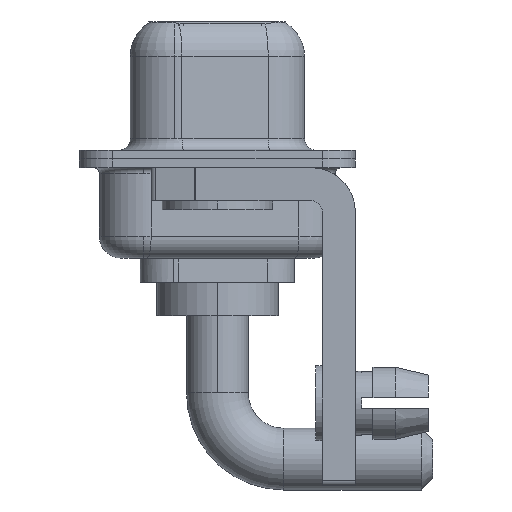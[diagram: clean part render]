
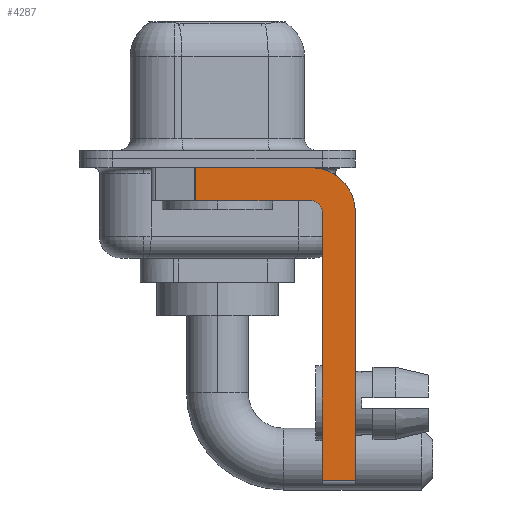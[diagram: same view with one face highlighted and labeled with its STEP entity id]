
A CAD part, left-side view. The second image highlights one B-rep face of the part: STEP entity #4287.
In plain terms, the highlighted planar face has unit normal (-1, 0, 0).
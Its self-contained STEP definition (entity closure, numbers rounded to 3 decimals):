
#157 = DIRECTION ( 'NONE',  ( -1., 0., 0. ) ) ;
#300 = DIRECTION ( 'NONE',  ( 0., -1., 0. ) ) ;
#726 = CARTESIAN_POINT ( 'NONE',  ( -2.9, 0.978, -1.9 ) ) ;
#1326 = ORIENTED_EDGE ( 'NONE', *, *, #11066, .F. ) ;
#1435 = EDGE_CURVE ( 'NONE', #13794, #10026, #7171, .T. ) ;
#1585 = EDGE_CURVE ( 'NONE', #13017, #10026, #4203, .T. ) ;
#1808 = DIRECTION ( 'NONE',  ( 1., 0., 0. ) ) ;
#1882 = EDGE_CURVE ( 'NONE', #11429, #8898, #6978, .T. ) ;
#1981 = CARTESIAN_POINT ( 'NONE',  ( -2.9, -4.75, -2.4 ) ) ;
#2211 = AXIS2_PLACEMENT_3D ( 'NONE', #14716, #1808, #3368 ) ;
#2222 = CIRCLE ( 'NONE', #2211, 2. ) ;
#2811 = DIRECTION ( 'NONE',  ( 0., 0., 1. ) ) ;
#2895 = CARTESIAN_POINT ( 'NONE',  ( -2.9, -4.25, -1.9 ) ) ;
#3368 = DIRECTION ( 'NONE',  ( 0., 0., -1. ) ) ;
#3976 = CARTESIAN_POINT ( 'NONE',  ( -2.9, -6.25, -2.4 ) ) ;
#4047 = DIRECTION ( 'NONE',  ( 0., 0., -1. ) ) ;
#4203 = LINE ( 'NONE', #12189, #13978 ) ;
#4283 = DIRECTION ( 'NONE',  ( 0., 0., -1. ) ) ;
#4287 = ADVANCED_FACE ( 'NONE', ( #6361 ), #8532, .F. ) ;
#4572 = CIRCLE ( 'NONE', #12906, 0.5 ) ;
#4833 = DIRECTION ( 'NONE',  ( 0., 1., 0. ) ) ;
#4939 = LINE ( 'NONE', #7006, #14163 ) ;
#4946 = ORIENTED_EDGE ( 'NONE', *, *, #11158, .F. ) ;
#4957 = ORIENTED_EDGE ( 'NONE', *, *, #8783, .F. ) ;
#4991 = ORIENTED_EDGE ( 'NONE', *, *, #1435, .F. ) ;
#5281 = AXIS2_PLACEMENT_3D ( 'NONE', #8834, #14218, #4283 ) ;
#5479 = EDGE_CURVE ( 'NONE', #8680, #8898, #11566, .T. ) ;
#6321 = EDGE_LOOP ( 'NONE', ( #4946, #8584, #10918, #7798, #4957, #13199, #4991, #1326 ) ) ;
#6361 = FACE_OUTER_BOUND ( 'NONE', #6321, .T. ) ;
#6978 = LINE ( 'NONE', #13871, #12560 ) ;
#7006 = CARTESIAN_POINT ( 'NONE',  ( -2.9, 3., -0.4 ) ) ;
#7130 = CARTESIAN_POINT ( 'NONE',  ( -2.9, 0.978, -1.9 ) ) ;
#7171 = LINE ( 'NONE', #3976, #7762 ) ;
#7762 = VECTOR ( 'NONE', #4047, 1000. ) ;
#7798 = ORIENTED_EDGE ( 'NONE', *, *, #8747, .F. ) ;
#8532 = PLANE ( 'NONE',  #5281 ) ;
#8584 = ORIENTED_EDGE ( 'NONE', *, *, #5479, .T. ) ;
#8680 = VERTEX_POINT ( 'NONE', #10447 ) ;
#8747 = EDGE_CURVE ( 'NONE', #11525, #11429, #4572, .T. ) ;
#8783 = EDGE_CURVE ( 'NONE', #13017, #11525, #10591, .T. ) ;
#8834 = CARTESIAN_POINT ( 'NONE',  ( -2.9, -4.25, -2.4 ) ) ;
#8898 = VERTEX_POINT ( 'NONE', #726 ) ;
#9259 = DIRECTION ( 'NONE',  ( 0., 0., 1. ) ) ;
#9473 = CARTESIAN_POINT ( 'NONE',  ( -2.9, -4.75, -14.8 ) ) ;
#9536 = VECTOR ( 'NONE', #2811, 1000. ) ;
#9962 = CARTESIAN_POINT ( 'NONE',  ( -2.9, -6.25, -2.4 ) ) ;
#10026 = VERTEX_POINT ( 'NONE', #11690 ) ;
#10447 = CARTESIAN_POINT ( 'NONE',  ( -2.9, 0.978, -0.4 ) ) ;
#10471 = VECTOR ( 'NONE', #10576, 1000. ) ;
#10576 = DIRECTION ( 'NONE',  ( 0., 0., -1. ) ) ;
#10591 = LINE ( 'NONE', #9473, #9536 ) ;
#10670 = CARTESIAN_POINT ( 'NONE',  ( -2.9, -4.25, -2.4 ) ) ;
#10918 = ORIENTED_EDGE ( 'NONE', *, *, #1882, .F. ) ;
#11066 = EDGE_CURVE ( 'NONE', #12362, #13794, #2222, .T. ) ;
#11158 = EDGE_CURVE ( 'NONE', #8680, #12362, #4939, .T. ) ;
#11425 = DIRECTION ( 'NONE',  ( 0., -1., 0. ) ) ;
#11429 = VERTEX_POINT ( 'NONE', #2895 ) ;
#11525 = VERTEX_POINT ( 'NONE', #1981 ) ;
#11566 = LINE ( 'NONE', #7130, #10471 ) ;
#11690 = CARTESIAN_POINT ( 'NONE',  ( -2.9, -6.25, -14.55 ) ) ;
#12189 = CARTESIAN_POINT ( 'NONE',  ( -2.9, -4.25, -14.55 ) ) ;
#12362 = VERTEX_POINT ( 'NONE', #14142 ) ;
#12560 = VECTOR ( 'NONE', #4833, 1000. ) ;
#12564 = CARTESIAN_POINT ( 'NONE',  ( -2.9, -4.75, -14.55 ) ) ;
#12906 = AXIS2_PLACEMENT_3D ( 'NONE', #10670, #157, #9259 ) ;
#13017 = VERTEX_POINT ( 'NONE', #12564 ) ;
#13199 = ORIENTED_EDGE ( 'NONE', *, *, #1585, .T. ) ;
#13794 = VERTEX_POINT ( 'NONE', #9962 ) ;
#13871 = CARTESIAN_POINT ( 'NONE',  ( -2.9, -4.25, -1.9 ) ) ;
#13978 = VECTOR ( 'NONE', #11425, 1000. ) ;
#14142 = CARTESIAN_POINT ( 'NONE',  ( -2.9, -4.25, -0.4 ) ) ;
#14163 = VECTOR ( 'NONE', #300, 1000. ) ;
#14218 = DIRECTION ( 'NONE',  ( 1., 0., 0. ) ) ;
#14716 = CARTESIAN_POINT ( 'NONE',  ( -2.9, -4.25, -2.4 ) ) ;
